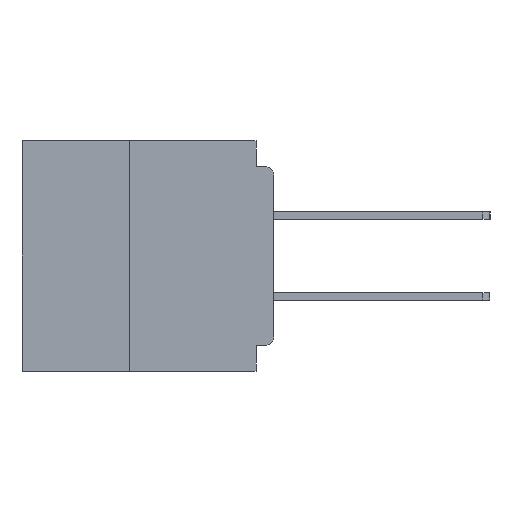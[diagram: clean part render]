
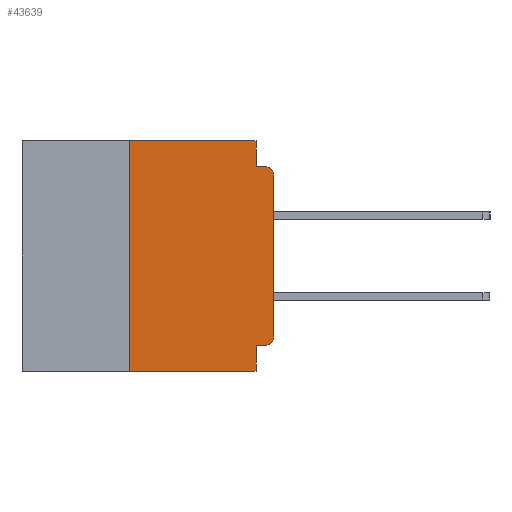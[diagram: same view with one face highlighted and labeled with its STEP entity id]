
A CAD part, left-side view. The second image highlights one B-rep face of the part: STEP entity #43639.
In plain terms, the highlighted planar face has unit normal (-1, 0, 0).
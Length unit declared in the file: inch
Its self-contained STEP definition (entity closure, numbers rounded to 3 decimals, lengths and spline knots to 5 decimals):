
#719 = DIRECTION ( 'NONE',  ( 1., 0., 0. ) ) ;
#993 = DIRECTION ( 'NONE',  ( -1., 0., 0. ) ) ;
#1859 = AXIS2_PLACEMENT_3D ( 'NONE', #24100, #993, #28027 ) ;
#1927 = ORIENTED_EDGE ( 'NONE', *, *, #47014, .F. ) ;
#2518 = LINE ( 'NONE', #14082, #41070 ) ;
#2657 = EDGE_LOOP ( 'NONE', ( #23004, #27365, #1927, #30391, #30817, #8992, #3057, #46173, #34056, #22592 ) ) ;
#3057 = ORIENTED_EDGE ( 'NONE', *, *, #33511, .T. ) ;
#3278 = VECTOR ( 'NONE', #15466, 39.37008 ) ;
#4378 = VERTEX_POINT ( 'NONE', #28788 ) ;
#5257 = EDGE_CURVE ( 'NONE', #41303, #28834, #9624, .T. ) ;
#5451 = LINE ( 'NONE', #24876, #15709 ) ;
#5707 = EDGE_CURVE ( 'NONE', #16210, #42989, #41507, .T. ) ;
#7019 = LINE ( 'NONE', #22354, #35383 ) ;
#7945 = VECTOR ( 'NONE', #15331, 39.37008 ) ;
#8064 = EDGE_CURVE ( 'NONE', #41303, #4378, #13547, .T. ) ;
#8302 = FACE_OUTER_BOUND ( 'NONE', #2657, .T. ) ;
#8731 = VERTEX_POINT ( 'NONE', #8908 ) ;
#8908 = CARTESIAN_POINT ( 'NONE',  ( 0., 0.031, 0. ) ) ;
#8968 = CARTESIAN_POINT ( 'NONE',  ( 0., 0.437, 0. ) ) ;
#8992 = ORIENTED_EDGE ( 'NONE', *, *, #47135, .F. ) ;
#9569 = DIRECTION ( 'NONE',  ( 0., 0., -1. ) ) ;
#9624 = CIRCLE ( 'NONE', #29660, 0.015 ) ;
#10193 = LINE ( 'NONE', #14737, #49854 ) ;
#10242 = VERTEX_POINT ( 'NONE', #37759 ) ;
#10355 = EDGE_CURVE ( 'NONE', #8731, #10242, #19414, .T. ) ;
#11458 = CARTESIAN_POINT ( 'NONE',  ( 0., 0.031, 0. ) ) ;
#11593 = CARTESIAN_POINT ( 'NONE',  ( 0., 0., -0.355 ) ) ;
#11630 = VERTEX_POINT ( 'NONE', #17411 ) ;
#12215 = PLANE ( 'NONE',  #44888 ) ;
#12834 = DIRECTION ( 'NONE',  ( 0., -1., 0. ) ) ;
#13547 = LINE ( 'NONE', #11593, #3278 ) ;
#14082 = CARTESIAN_POINT ( 'NONE',  ( 0., 0., -0.045 ) ) ;
#14737 = CARTESIAN_POINT ( 'NONE',  ( 0., 0.25, -0.4 ) ) ;
#15092 = VECTOR ( 'NONE', #12834, 39.37008 ) ;
#15331 = DIRECTION ( 'NONE',  ( 0., 0., -1. ) ) ;
#15466 = DIRECTION ( 'NONE',  ( 0., 1., 0. ) ) ;
#15492 = VECTOR ( 'NONE', #9569, 39.37008 ) ;
#15709 = VECTOR ( 'NONE', #20845, 39.37008 ) ;
#16210 = VERTEX_POINT ( 'NONE', #44618 ) ;
#17411 = CARTESIAN_POINT ( 'NONE',  ( 0., 0.25, 0. ) ) ;
#18388 = VERTEX_POINT ( 'NONE', #34982 ) ;
#19414 = LINE ( 'NONE', #11458, #7945 ) ;
#20845 = DIRECTION ( 'NONE',  ( 0., 0., 1. ) ) ;
#21758 = VERTEX_POINT ( 'NONE', #38918 ) ;
#22354 = CARTESIAN_POINT ( 'NONE',  ( 0., 0.437, -0.4 ) ) ;
#22421 = DIRECTION ( 'NONE',  ( -1., 0., 0. ) ) ;
#22592 = ORIENTED_EDGE ( 'NONE', *, *, #5257, .T. ) ;
#22645 = EDGE_CURVE ( 'NONE', #28834, #16210, #5451, .T. ) ;
#23004 = ORIENTED_EDGE ( 'NONE', *, *, #22645, .T. ) ;
#23829 = CARTESIAN_POINT ( 'NONE',  ( 0., 0.437, 0. ) ) ;
#24100 = CARTESIAN_POINT ( 'NONE',  ( 0., 0.015, -0.06 ) ) ;
#24876 = CARTESIAN_POINT ( 'NONE',  ( 0., 0., 0. ) ) ;
#27365 = ORIENTED_EDGE ( 'NONE', *, *, #5707, .T. ) ;
#27754 = DIRECTION ( 'NONE',  ( 0., 0., -1. ) ) ;
#28027 = DIRECTION ( 'NONE',  ( 0., 0., -1. ) ) ;
#28788 = CARTESIAN_POINT ( 'NONE',  ( 0., 0.031, -0.355 ) ) ;
#28834 = VERTEX_POINT ( 'NONE', #39457 ) ;
#29660 = AXIS2_PLACEMENT_3D ( 'NONE', #45398, #22421, #49248 ) ;
#30391 = ORIENTED_EDGE ( 'NONE', *, *, #10355, .F. ) ;
#30658 = EDGE_CURVE ( 'NONE', #11630, #8731, #44537, .T. ) ;
#30817 = ORIENTED_EDGE ( 'NONE', *, *, #30658, .F. ) ;
#33293 = EDGE_CURVE ( 'NONE', #4378, #21758, #46131, .T. ) ;
#33511 = EDGE_CURVE ( 'NONE', #18388, #21758, #7019, .T. ) ;
#34056 = ORIENTED_EDGE ( 'NONE', *, *, #8064, .F. ) ;
#34982 = CARTESIAN_POINT ( 'NONE',  ( 0., 0.25, -0.4 ) ) ;
#35383 = VECTOR ( 'NONE', #37683, 39.37008 ) ;
#35652 = CARTESIAN_POINT ( 'NONE',  ( 0., 0.015, -0.355 ) ) ;
#37683 = DIRECTION ( 'NONE',  ( 0., -1., 0. ) ) ;
#37759 = CARTESIAN_POINT ( 'NONE',  ( 0., 0.031, -0.045 ) ) ;
#38918 = CARTESIAN_POINT ( 'NONE',  ( 0., 0.031, -0.4 ) ) ;
#39347 = CARTESIAN_POINT ( 'NONE',  ( 0., 0.015, -0.045 ) ) ;
#39457 = CARTESIAN_POINT ( 'NONE',  ( 0., 0., -0.34 ) ) ;
#41015 = DIRECTION ( 'NONE',  ( 0., -1., 0. ) ) ;
#41070 = VECTOR ( 'NONE', #41015, 39.37008 ) ;
#41303 = VERTEX_POINT ( 'NONE', #35652 ) ;
#41507 = CIRCLE ( 'NONE', #1859, 0.015 ) ;
#41678 = DIRECTION ( 'NONE',  ( 0., 0., 1. ) ) ;
#42989 = VERTEX_POINT ( 'NONE', #39347 ) ;
#43639 = ADVANCED_FACE ( 'NONE', ( #8302 ), #12215, .F. ) ;
#44537 = LINE ( 'NONE', #8968, #15092 ) ;
#44618 = CARTESIAN_POINT ( 'NONE',  ( 0., 0., -0.06 ) ) ;
#44888 = AXIS2_PLACEMENT_3D ( 'NONE', #23829, #719, #27754 ) ;
#45398 = CARTESIAN_POINT ( 'NONE',  ( 0., 0.015, -0.34 ) ) ;
#46131 = LINE ( 'NONE', #47845, #15492 ) ;
#46173 = ORIENTED_EDGE ( 'NONE', *, *, #33293, .F. ) ;
#47014 = EDGE_CURVE ( 'NONE', #10242, #42989, #2518, .T. ) ;
#47135 = EDGE_CURVE ( 'NONE', #18388, #11630, #10193, .T. ) ;
#47845 = CARTESIAN_POINT ( 'NONE',  ( 0., 0.031, -0.4 ) ) ;
#49248 = DIRECTION ( 'NONE',  ( 0., 0., -1. ) ) ;
#49854 = VECTOR ( 'NONE', #41678, 39.37008 ) ;
